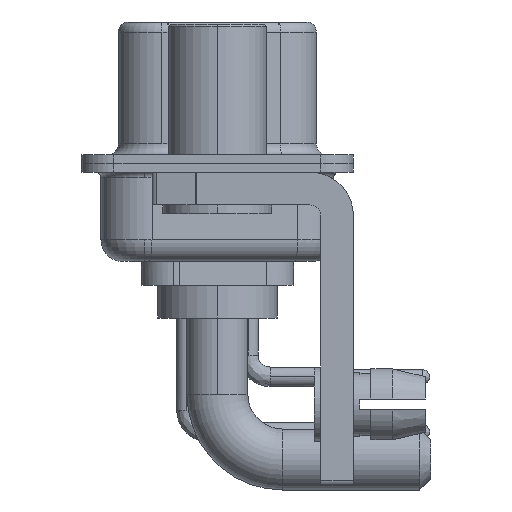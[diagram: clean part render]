
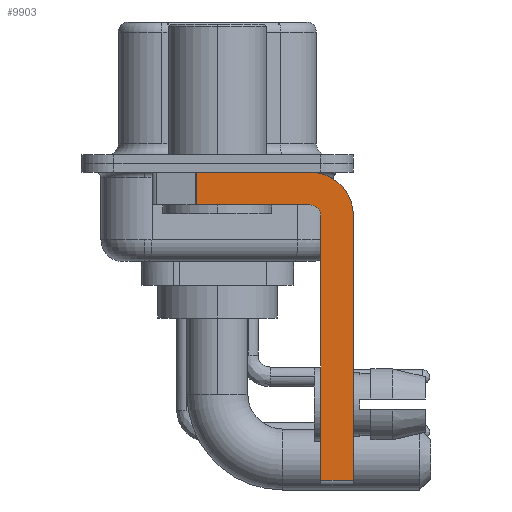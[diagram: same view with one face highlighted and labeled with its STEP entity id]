
A CAD part, left-side view. The second image highlights one B-rep face of the part: STEP entity #9903.
In plain terms, the highlighted planar face has unit normal (-1, 0, 0).
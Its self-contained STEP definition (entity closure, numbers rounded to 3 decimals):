
#1149 = VERTEX_POINT ( 'NONE', #24994 ) ;
#1650 = VERTEX_POINT ( 'NONE', #24566 ) ;
#2308 = DIRECTION ( 'NONE',  ( 0., 0., 1. ) ) ;
#2503 = CARTESIAN_POINT ( 'NONE',  ( -2.9, -6.25, -14.55 ) ) ;
#2913 = DIRECTION ( 'NONE',  ( 1., 0., 0. ) ) ;
#3129 = VECTOR ( 'NONE', #13497, 1000. ) ;
#3331 = CARTESIAN_POINT ( 'NONE',  ( -2.9, -4.25, -2.4 ) ) ;
#3549 = ORIENTED_EDGE ( 'NONE', *, *, #20440, .F. ) ;
#3876 = EDGE_CURVE ( 'NONE', #11489, #16978, #14716, .T. ) ;
#4418 = LINE ( 'NONE', #13595, #11891 ) ;
#5698 = DIRECTION ( 'NONE',  ( 0., 1., 0. ) ) ;
#5923 = VECTOR ( 'NONE', #5698, 1000. ) ;
#6204 = DIRECTION ( 'NONE',  ( 0., 0., -1. ) ) ;
#6535 = VERTEX_POINT ( 'NONE', #17483 ) ;
#6793 = VECTOR ( 'NONE', #19238, 1000. ) ;
#7524 = CARTESIAN_POINT ( 'NONE',  ( -2.9, 0.978, -0.4 ) ) ;
#8385 = DIRECTION ( 'NONE',  ( 0., -1., 0. ) ) ;
#8540 = LINE ( 'NONE', #29464, #3129 ) ;
#8737 = LINE ( 'NONE', #18204, #21221 ) ;
#9494 = DIRECTION ( 'NONE',  ( -1., 0., 0. ) ) ;
#9513 = VECTOR ( 'NONE', #8385, 1000. ) ;
#9903 = ADVANCED_FACE ( 'NONE', ( #22754 ), #19882, .F. ) ;
#10192 = LINE ( 'NONE', #26327, #5923 ) ;
#11489 = VERTEX_POINT ( 'NONE', #28910 ) ;
#11516 = ORIENTED_EDGE ( 'NONE', *, *, #15989, .F. ) ;
#11546 = AXIS2_PLACEMENT_3D ( 'NONE', #3331, #9494, #28019 ) ;
#11858 = VERTEX_POINT ( 'NONE', #12614 ) ;
#11891 = VECTOR ( 'NONE', #2308, 1000. ) ;
#12095 = DIRECTION ( 'NONE',  ( 0., 0., -1. ) ) ;
#12614 = CARTESIAN_POINT ( 'NONE',  ( -2.9, -4.25, -1.9 ) ) ;
#13150 = AXIS2_PLACEMENT_3D ( 'NONE', #22128, #2913, #12095 ) ;
#13233 = CARTESIAN_POINT ( 'NONE',  ( -2.9, 0.978, -1.9 ) ) ;
#13497 = DIRECTION ( 'NONE',  ( 0., -1., 0. ) ) ;
#13595 = CARTESIAN_POINT ( 'NONE',  ( -2.9, -4.75, -14.8 ) ) ;
#14578 = EDGE_CURVE ( 'NONE', #19819, #16319, #8737, .T. ) ;
#14716 = LINE ( 'NONE', #24365, #9513 ) ;
#15568 = ORIENTED_EDGE ( 'NONE', *, *, #21213, .F. ) ;
#15803 = EDGE_LOOP ( 'NONE', ( #25712, #21024, #3549, #11516, #22489, #29363, #23239, #15568 ) ) ;
#15989 = EDGE_CURVE ( 'NONE', #1149, #11858, #22614, .T. ) ;
#16319 = VERTEX_POINT ( 'NONE', #13233 ) ;
#16978 = VERTEX_POINT ( 'NONE', #2503 ) ;
#17483 = CARTESIAN_POINT ( 'NONE',  ( -2.9, -6.25, -2.4 ) ) ;
#17611 = CARTESIAN_POINT ( 'NONE',  ( -2.9, -4.25, -2.4 ) ) ;
#18204 = CARTESIAN_POINT ( 'NONE',  ( -2.9, 0.978, -1.9 ) ) ;
#18907 = CIRCLE ( 'NONE', #13150, 2. ) ;
#19238 = DIRECTION ( 'NONE',  ( 0., 0., -1. ) ) ;
#19819 = VERTEX_POINT ( 'NONE', #7524 ) ;
#19882 = PLANE ( 'NONE',  #23782 ) ;
#20440 = EDGE_CURVE ( 'NONE', #11858, #16319, #10192, .T. ) ;
#21024 = ORIENTED_EDGE ( 'NONE', *, *, #14578, .T. ) ;
#21213 = EDGE_CURVE ( 'NONE', #1650, #6535, #18907, .T. ) ;
#21221 = VECTOR ( 'NONE', #29678, 1000. ) ;
#21970 = EDGE_CURVE ( 'NONE', #19819, #1650, #8540, .T. ) ;
#22128 = CARTESIAN_POINT ( 'NONE',  ( -2.9, -4.25, -2.4 ) ) ;
#22489 = ORIENTED_EDGE ( 'NONE', *, *, #26119, .F. ) ;
#22614 = CIRCLE ( 'NONE', #11546, 0.5 ) ;
#22754 = FACE_OUTER_BOUND ( 'NONE', #15803, .T. ) ;
#23239 = ORIENTED_EDGE ( 'NONE', *, *, #26791, .F. ) ;
#23782 = AXIS2_PLACEMENT_3D ( 'NONE', #17611, #26830, #6204 ) ;
#23786 = CARTESIAN_POINT ( 'NONE',  ( -2.9, -6.25, -2.4 ) ) ;
#24365 = CARTESIAN_POINT ( 'NONE',  ( -2.9, -4.25, -14.55 ) ) ;
#24566 = CARTESIAN_POINT ( 'NONE',  ( -2.9, -4.25, -0.4 ) ) ;
#24994 = CARTESIAN_POINT ( 'NONE',  ( -2.9, -4.75, -2.4 ) ) ;
#25712 = ORIENTED_EDGE ( 'NONE', *, *, #21970, .F. ) ;
#26054 = LINE ( 'NONE', #23786, #6793 ) ;
#26119 = EDGE_CURVE ( 'NONE', #11489, #1149, #4418, .T. ) ;
#26327 = CARTESIAN_POINT ( 'NONE',  ( -2.9, -4.25, -1.9 ) ) ;
#26791 = EDGE_CURVE ( 'NONE', #6535, #16978, #26054, .T. ) ;
#26830 = DIRECTION ( 'NONE',  ( 1., 0., 0. ) ) ;
#28019 = DIRECTION ( 'NONE',  ( 0., 0., 1. ) ) ;
#28910 = CARTESIAN_POINT ( 'NONE',  ( -2.9, -4.75, -14.55 ) ) ;
#29363 = ORIENTED_EDGE ( 'NONE', *, *, #3876, .T. ) ;
#29464 = CARTESIAN_POINT ( 'NONE',  ( -2.9, 3., -0.4 ) ) ;
#29678 = DIRECTION ( 'NONE',  ( 0., 0., -1. ) ) ;
